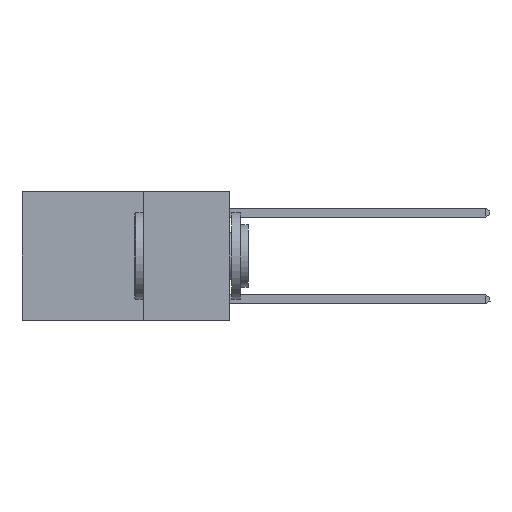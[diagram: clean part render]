
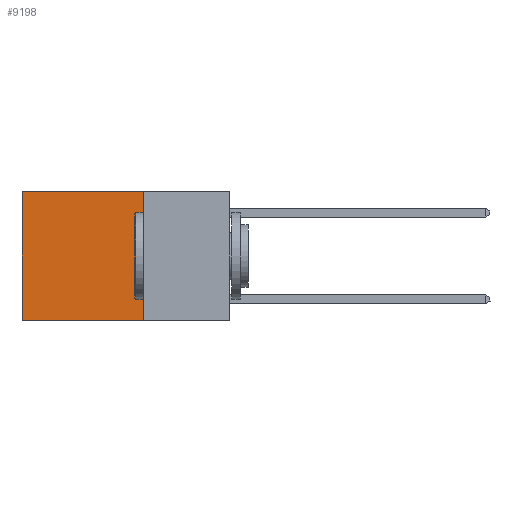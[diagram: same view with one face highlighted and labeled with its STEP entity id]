
A CAD part, left-side view. The second image highlights one B-rep face of the part: STEP entity #9198.
In plain terms, the highlighted planar face has unit normal (-1, 0, 0).
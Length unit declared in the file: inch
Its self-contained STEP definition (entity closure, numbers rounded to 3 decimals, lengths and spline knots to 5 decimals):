
#215 = FACE_OUTER_BOUND ( 'NONE', #3294, .T. ) ;
#1442 = VECTOR ( 'NONE', #10272, 39.37008 ) ;
#1506 = CARTESIAN_POINT ( 'NONE',  ( 0.2625, 0.6, -0.37 ) ) ;
#1953 = CARTESIAN_POINT ( 'NONE',  ( 0.2625, 0.25, 0. ) ) ;
#2803 = CARTESIAN_POINT ( 'NONE',  ( 0.2625, 0.6, 0. ) ) ;
#3294 = EDGE_LOOP ( 'NONE', ( #9188, #10182, #10427, #3383 ) ) ;
#3383 = ORIENTED_EDGE ( 'NONE', *, *, #9369, .T. ) ;
#3413 = DIRECTION ( 'NONE',  ( 0., 0., -1. ) ) ;
#3665 = CARTESIAN_POINT ( 'NONE',  ( 0.2625, 0.25, 0. ) ) ;
#4227 = VECTOR ( 'NONE', #8609, 39.37008 ) ;
#4667 = VERTEX_POINT ( 'NONE', #8285 ) ;
#5129 = LINE ( 'NONE', #2803, #4227 ) ;
#6187 = VERTEX_POINT ( 'NONE', #17360 ) ;
#6221 = PLANE ( 'NONE',  #11287 ) ;
#8285 = CARTESIAN_POINT ( 'NONE',  ( 0.2625, 0.6, 0. ) ) ;
#8295 = EDGE_CURVE ( 'NONE', #4667, #18084, #5129, .T. ) ;
#8405 = EDGE_CURVE ( 'NONE', #11288, #18084, #9639, .T. ) ;
#8609 = DIRECTION ( 'NONE',  ( 0., 0., -1. ) ) ;
#9165 = LINE ( 'NONE', #3665, #16262 ) ;
#9188 = ORIENTED_EDGE ( 'NONE', *, *, #8295, .T. ) ;
#9198 = ADVANCED_FACE ( 'NONE', ( #215 ), #6221, .F. ) ;
#9369 = EDGE_CURVE ( 'NONE', #6187, #4667, #9165, .T. ) ;
#9639 = LINE ( 'NONE', #15908, #1442 ) ;
#9955 = CARTESIAN_POINT ( 'NONE',  ( 0.2625, 0.25, 0. ) ) ;
#10182 = ORIENTED_EDGE ( 'NONE', *, *, #8405, .F. ) ;
#10272 = DIRECTION ( 'NONE',  ( 0., 1., 0. ) ) ;
#10427 = ORIENTED_EDGE ( 'NONE', *, *, #15124, .F. ) ;
#11287 = AXIS2_PLACEMENT_3D ( 'NONE', #1953, #12024, #3413 ) ;
#11288 = VERTEX_POINT ( 'NONE', #18694 ) ;
#11368 = DIRECTION ( 'NONE',  ( 0., 0., -1. ) ) ;
#12024 = DIRECTION ( 'NONE',  ( 1., 0., 0. ) ) ;
#13297 = VECTOR ( 'NONE', #11368, 39.37008 ) ;
#14203 = LINE ( 'NONE', #9955, #13297 ) ;
#15124 = EDGE_CURVE ( 'NONE', #6187, #11288, #14203, .T. ) ;
#15908 = CARTESIAN_POINT ( 'NONE',  ( 0.2625, 0.25, -0.37 ) ) ;
#16262 = VECTOR ( 'NONE', #16644, 39.37008 ) ;
#16644 = DIRECTION ( 'NONE',  ( 0., 1., 0. ) ) ;
#17360 = CARTESIAN_POINT ( 'NONE',  ( 0.2625, 0.25, 0. ) ) ;
#18084 = VERTEX_POINT ( 'NONE', #1506 ) ;
#18694 = CARTESIAN_POINT ( 'NONE',  ( 0.2625, 0.25, -0.37 ) ) ;
